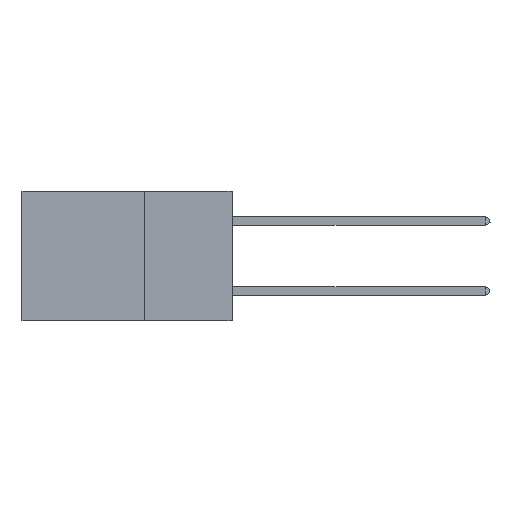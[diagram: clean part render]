
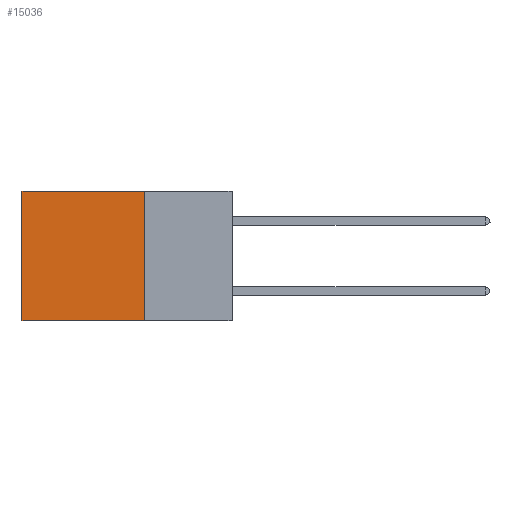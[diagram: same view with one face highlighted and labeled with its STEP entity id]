
A CAD part, left-side view. The second image highlights one B-rep face of the part: STEP entity #15036.
In plain terms, the highlighted planar face has unit normal (-1, 0, 0).
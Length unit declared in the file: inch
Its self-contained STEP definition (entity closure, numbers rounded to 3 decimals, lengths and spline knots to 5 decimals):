
#1091 = DIRECTION ( 'NONE',  ( 0., 0., -1. ) ) ;
#1875 = FACE_OUTER_BOUND ( 'NONE', #37114, .T. ) ;
#3276 = EDGE_CURVE ( 'NONE', #29907, #19200, #29236, .T. ) ;
#4127 = CARTESIAN_POINT ( 'NONE',  ( 0.2875, 0.6, 0. ) ) ;
#5185 = CARTESIAN_POINT ( 'NONE',  ( 0.2875, 0.25, 0. ) ) ;
#8521 = DIRECTION ( 'NONE',  ( 0., 0., -1. ) ) ;
#8998 = VERTEX_POINT ( 'NONE', #4127 ) ;
#13254 = VECTOR ( 'NONE', #8521, 39.37008 ) ;
#13949 = DIRECTION ( 'NONE',  ( 1., 0., 0. ) ) ;
#14362 = CARTESIAN_POINT ( 'NONE',  ( 0.2875, 0.25, 0. ) ) ;
#15036 = ADVANCED_FACE ( 'NONE', ( #1875 ), #28844, .F. ) ;
#16043 = CARTESIAN_POINT ( 'NONE',  ( 0.2875, 0.25, 0. ) ) ;
#16633 = LINE ( 'NONE', #16043, #22770 ) ;
#16964 = CARTESIAN_POINT ( 'NONE',  ( 0.2875, 0.25, 0. ) ) ;
#17154 = DIRECTION ( 'NONE',  ( 0., 1., 0. ) ) ;
#18406 = CARTESIAN_POINT ( 'NONE',  ( 0.2875, 0.25, -0.37 ) ) ;
#19200 = VERTEX_POINT ( 'NONE', #39204 ) ;
#19400 = LINE ( 'NONE', #31684, #38621 ) ;
#20487 = VERTEX_POINT ( 'NONE', #5185 ) ;
#21776 = ORIENTED_EDGE ( 'NONE', *, *, #24109, .T. ) ;
#22770 = VECTOR ( 'NONE', #25490, 39.37008 ) ;
#23410 = LINE ( 'NONE', #14362, #13254 ) ;
#24109 = EDGE_CURVE ( 'NONE', #8998, #19200, #19400, .T. ) ;
#25490 = DIRECTION ( 'NONE',  ( 0., 1., 0. ) ) ;
#28844 = PLANE ( 'NONE',  #37696 ) ;
#29236 = LINE ( 'NONE', #39066, #34739 ) ;
#29623 = EDGE_CURVE ( 'NONE', #20487, #8998, #16633, .T. ) ;
#29907 = VERTEX_POINT ( 'NONE', #18406 ) ;
#31632 = EDGE_CURVE ( 'NONE', #20487, #29907, #23410, .T. ) ;
#31684 = CARTESIAN_POINT ( 'NONE',  ( 0.2875, 0.6, 0. ) ) ;
#32948 = ORIENTED_EDGE ( 'NONE', *, *, #3276, .F. ) ;
#33570 = ORIENTED_EDGE ( 'NONE', *, *, #29623, .T. ) ;
#34676 = ORIENTED_EDGE ( 'NONE', *, *, #31632, .F. ) ;
#34739 = VECTOR ( 'NONE', #17154, 39.37008 ) ;
#35869 = DIRECTION ( 'NONE',  ( 0., 0., -1. ) ) ;
#37114 = EDGE_LOOP ( 'NONE', ( #21776, #32948, #34676, #33570 ) ) ;
#37696 = AXIS2_PLACEMENT_3D ( 'NONE', #16964, #13949, #1091 ) ;
#38621 = VECTOR ( 'NONE', #35869, 39.37008 ) ;
#39066 = CARTESIAN_POINT ( 'NONE',  ( 0.2875, 0.25, -0.37 ) ) ;
#39204 = CARTESIAN_POINT ( 'NONE',  ( 0.2875, 0.6, -0.37 ) ) ;
